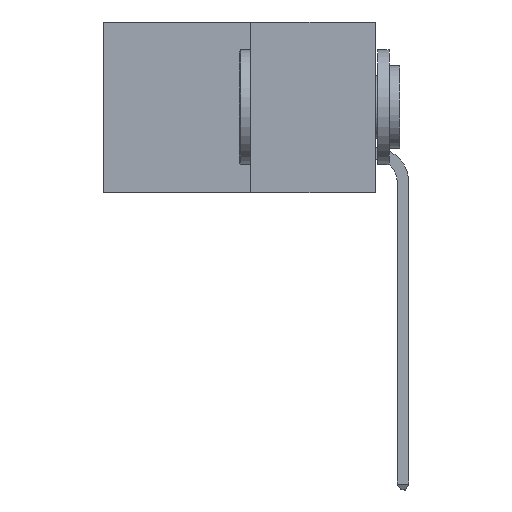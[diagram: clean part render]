
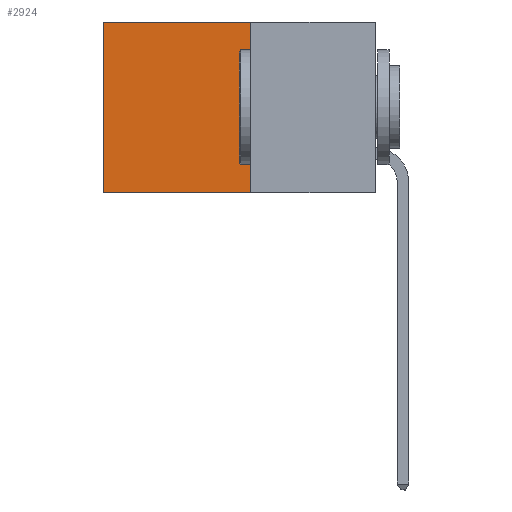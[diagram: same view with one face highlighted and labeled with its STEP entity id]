
A CAD part, left-side view. The second image highlights one B-rep face of the part: STEP entity #2924.
In plain terms, the highlighted planar face has unit normal (-1, 0, 0).
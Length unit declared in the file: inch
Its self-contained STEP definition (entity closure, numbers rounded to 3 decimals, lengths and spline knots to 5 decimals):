
#159 = CARTESIAN_POINT ( 'NONE',  ( 0.277, 0.59, 0. ) ) ;
#841 = EDGE_CURVE ( 'NONE', #21423, #23710, #3651, .T. ) ;
#1770 = DIRECTION ( 'NONE',  ( 0., 1., 0. ) ) ;
#1775 = ORIENTED_EDGE ( 'NONE', *, *, #13838, .F. ) ;
#1951 = VECTOR ( 'NONE', #24186, 39.37008 ) ;
#2335 = CARTESIAN_POINT ( 'NONE',  ( 0.277, 0.59, -0.37 ) ) ;
#2924 = ADVANCED_FACE ( 'NONE', ( #12966 ), #13269, .F. ) ;
#3063 = DIRECTION ( 'NONE',  ( 0., 0., -1. ) ) ;
#3574 = DIRECTION ( 'NONE',  ( 0., 0., -1. ) ) ;
#3651 = LINE ( 'NONE', #2335, #16954 ) ;
#3887 = AXIS2_PLACEMENT_3D ( 'NONE', #8974, #4517, #3574 ) ;
#4517 = DIRECTION ( 'NONE',  ( 1., 0., 0. ) ) ;
#4823 = CARTESIAN_POINT ( 'NONE',  ( 0.277, 0.27, -0.37 ) ) ;
#6542 = CARTESIAN_POINT ( 'NONE',  ( 0.277, 0.27, -0.37 ) ) ;
#7490 = CARTESIAN_POINT ( 'NONE',  ( 0.277, 0.27, 0. ) ) ;
#8974 = CARTESIAN_POINT ( 'NONE',  ( 0.277, 0.27, -0.37 ) ) ;
#8991 = VECTOR ( 'NONE', #1770, 39.37008 ) ;
#9535 = ORIENTED_EDGE ( 'NONE', *, *, #20392, .F. ) ;
#9801 = CARTESIAN_POINT ( 'NONE',  ( 0.277, 0.27, 0. ) ) ;
#10054 = VERTEX_POINT ( 'NONE', #4823 ) ;
#10536 = ORIENTED_EDGE ( 'NONE', *, *, #841, .T. ) ;
#12102 = ORIENTED_EDGE ( 'NONE', *, *, #13497, .T. ) ;
#12966 = FACE_OUTER_BOUND ( 'NONE', #13095, .T. ) ;
#13095 = EDGE_LOOP ( 'NONE', ( #10536, #1775, #9535, #12102 ) ) ;
#13269 = PLANE ( 'NONE',  #3887 ) ;
#13497 = EDGE_CURVE ( 'NONE', #14903, #21423, #19023, .T. ) ;
#13838 = EDGE_CURVE ( 'NONE', #10054, #23710, #16345, .T. ) ;
#14131 = DIRECTION ( 'NONE',  ( 0., 1., 0. ) ) ;
#14394 = CARTESIAN_POINT ( 'NONE',  ( 0.277, 0.59, -0.37 ) ) ;
#14903 = VERTEX_POINT ( 'NONE', #9801 ) ;
#16345 = LINE ( 'NONE', #6542, #20194 ) ;
#16954 = VECTOR ( 'NONE', #3063, 39.37008 ) ;
#17010 = LINE ( 'NONE', #22317, #1951 ) ;
#19023 = LINE ( 'NONE', #7490, #8991 ) ;
#20194 = VECTOR ( 'NONE', #14131, 39.37008 ) ;
#20392 = EDGE_CURVE ( 'NONE', #14903, #10054, #17010, .T. ) ;
#21423 = VERTEX_POINT ( 'NONE', #159 ) ;
#22317 = CARTESIAN_POINT ( 'NONE',  ( 0.277, 0.27, -0.37 ) ) ;
#23710 = VERTEX_POINT ( 'NONE', #14394 ) ;
#24186 = DIRECTION ( 'NONE',  ( 0., 0., -1. ) ) ;
